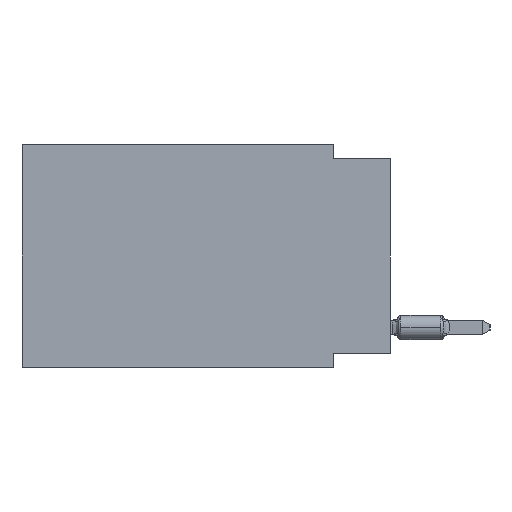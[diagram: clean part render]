
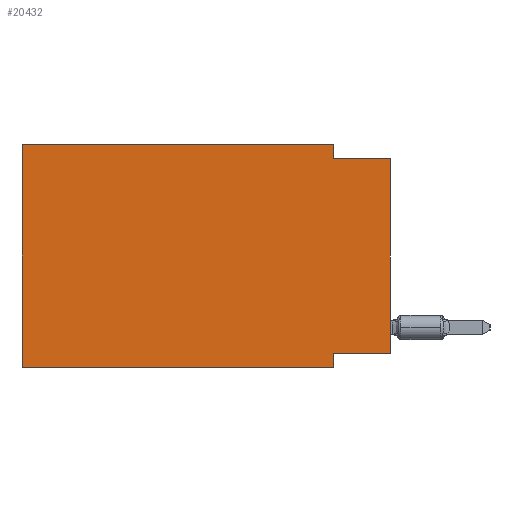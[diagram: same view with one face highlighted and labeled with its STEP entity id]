
A CAD part, left-side view. The second image highlights one B-rep face of the part: STEP entity #20432.
In plain terms, the highlighted planar face has unit normal (-1, 0, 0).
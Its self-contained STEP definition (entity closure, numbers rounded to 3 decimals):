
#484 = CARTESIAN_POINT ( 'NONE',  ( 0., 16.383, -9.906 ) ) ;
#2166 = DIRECTION ( 'NONE',  ( 0., 0., -1. ) ) ;
#3325 = CARTESIAN_POINT ( 'NONE',  ( 0., 16.383, 0. ) ) ;
#4135 = EDGE_CURVE ( 'NONE', #4284, #15853, #20141, .T. ) ;
#4284 = VERTEX_POINT ( 'NONE', #21004 ) ;
#4484 = EDGE_CURVE ( 'NONE', #38869, #15853, #22930, .T. ) ;
#4904 = DIRECTION ( 'NONE',  ( 0., -1., 0. ) ) ;
#5842 = LINE ( 'NONE', #32769, #40198 ) ;
#6031 = CARTESIAN_POINT ( 'NONE',  ( 0., 0., 0. ) ) ;
#6186 = EDGE_CURVE ( 'NONE', #25286, #36546, #24695, .T. ) ;
#8656 = EDGE_CURVE ( 'NONE', #4284, #18768, #24942, .T. ) ;
#8697 = ORIENTED_EDGE ( 'NONE', *, *, #13671, .F. ) ;
#9218 = LINE ( 'NONE', #25545, #32437 ) ;
#10421 = EDGE_CURVE ( 'NONE', #36546, #38869, #5842, .T. ) ;
#11558 = DIRECTION ( 'NONE',  ( 0., 0., 1. ) ) ;
#13671 = EDGE_CURVE ( 'NONE', #28599, #25286, #28929, .T. ) ;
#14199 = ORIENTED_EDGE ( 'NONE', *, *, #6186, .F. ) ;
#14253 = ORIENTED_EDGE ( 'NONE', *, *, #4484, .F. ) ;
#15496 = VECTOR ( 'NONE', #11558, 1000. ) ;
#15730 = VECTOR ( 'NONE', #42864, 1000. ) ;
#15853 = VERTEX_POINT ( 'NONE', #18984 ) ;
#16153 = DIRECTION ( 'NONE',  ( 0., 0., -1. ) ) ;
#17315 = ORIENTED_EDGE ( 'NONE', *, *, #4135, .T. ) ;
#17708 = AXIS2_PLACEMENT_3D ( 'NONE', #32242, #25739, #16153 ) ;
#17948 = VECTOR ( 'NONE', #4904, 1000. ) ;
#18025 = VECTOR ( 'NONE', #27761, 1000. ) ;
#18768 = VERTEX_POINT ( 'NONE', #22913 ) ;
#18984 = CARTESIAN_POINT ( 'NONE',  ( 0., 0., -0.635 ) ) ;
#19824 = ORIENTED_EDGE ( 'NONE', *, *, #25355, .T. ) ;
#20141 = LINE ( 'NONE', #6031, #30969 ) ;
#20432 = ADVANCED_FACE ( 'NONE', ( #32030 ), #35481, .F. ) ;
#20883 = VERTEX_POINT ( 'NONE', #36068 ) ;
#21004 = CARTESIAN_POINT ( 'NONE',  ( 0., 0., -9.271 ) ) ;
#21247 = ORIENTED_EDGE ( 'NONE', *, *, #8656, .F. ) ;
#22913 = CARTESIAN_POINT ( 'NONE',  ( 0., 2.54, -9.271 ) ) ;
#22930 = LINE ( 'NONE', #35724, #15730 ) ;
#23561 = EDGE_CURVE ( 'NONE', #18768, #20883, #9218, .T. ) ;
#24695 = LINE ( 'NONE', #34449, #17948 ) ;
#24942 = LINE ( 'NONE', #37495, #18025 ) ;
#25286 = VERTEX_POINT ( 'NONE', #3325 ) ;
#25355 = EDGE_CURVE ( 'NONE', #28599, #20883, #30237, .T. ) ;
#25545 = CARTESIAN_POINT ( 'NONE',  ( 0., 2.54, -9.906 ) ) ;
#25739 = DIRECTION ( 'NONE',  ( 1., 0., 0. ) ) ;
#26247 = DIRECTION ( 'NONE',  ( 0., 0., 1. ) ) ;
#26985 = VECTOR ( 'NONE', #30663, 1000. ) ;
#27761 = DIRECTION ( 'NONE',  ( 0., 1., 0. ) ) ;
#28080 = CARTESIAN_POINT ( 'NONE',  ( 0., 16.383, 0. ) ) ;
#28599 = VERTEX_POINT ( 'NONE', #38948 ) ;
#28929 = LINE ( 'NONE', #28080, #15496 ) ;
#28994 = DIRECTION ( 'NONE',  ( 0., 0., -1. ) ) ;
#29175 = CARTESIAN_POINT ( 'NONE',  ( 0., 2.54, -0.635 ) ) ;
#30237 = LINE ( 'NONE', #484, #26985 ) ;
#30650 = CARTESIAN_POINT ( 'NONE',  ( 0., 2.54, 0. ) ) ;
#30663 = DIRECTION ( 'NONE',  ( 0., -1., 0. ) ) ;
#30969 = VECTOR ( 'NONE', #26247, 1000. ) ;
#32030 = FACE_OUTER_BOUND ( 'NONE', #40411, .T. ) ;
#32242 = CARTESIAN_POINT ( 'NONE',  ( 0., 16.383, 0. ) ) ;
#32437 = VECTOR ( 'NONE', #28994, 1000. ) ;
#32769 = CARTESIAN_POINT ( 'NONE',  ( 0., 2.54, 0. ) ) ;
#34449 = CARTESIAN_POINT ( 'NONE',  ( 0., 16.383, 0. ) ) ;
#35481 = PLANE ( 'NONE',  #17708 ) ;
#35724 = CARTESIAN_POINT ( 'NONE',  ( 0., 0., -0.635 ) ) ;
#35858 = ORIENTED_EDGE ( 'NONE', *, *, #10421, .F. ) ;
#36068 = CARTESIAN_POINT ( 'NONE',  ( 0., 2.54, -9.906 ) ) ;
#36546 = VERTEX_POINT ( 'NONE', #30650 ) ;
#36670 = ORIENTED_EDGE ( 'NONE', *, *, #23561, .F. ) ;
#37495 = CARTESIAN_POINT ( 'NONE',  ( 0., 0., -9.271 ) ) ;
#38869 = VERTEX_POINT ( 'NONE', #29175 ) ;
#38948 = CARTESIAN_POINT ( 'NONE',  ( 0., 16.383, -9.906 ) ) ;
#40198 = VECTOR ( 'NONE', #2166, 1000. ) ;
#40411 = EDGE_LOOP ( 'NONE', ( #17315, #14253, #35858, #14199, #8697, #19824, #36670, #21247 ) ) ;
#42864 = DIRECTION ( 'NONE',  ( 0., -1., 0. ) ) ;
